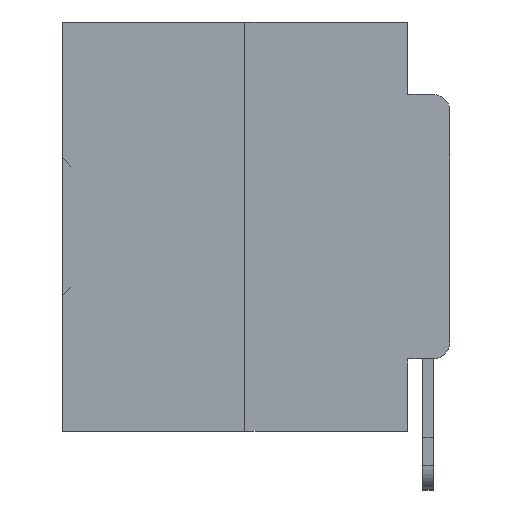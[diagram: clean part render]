
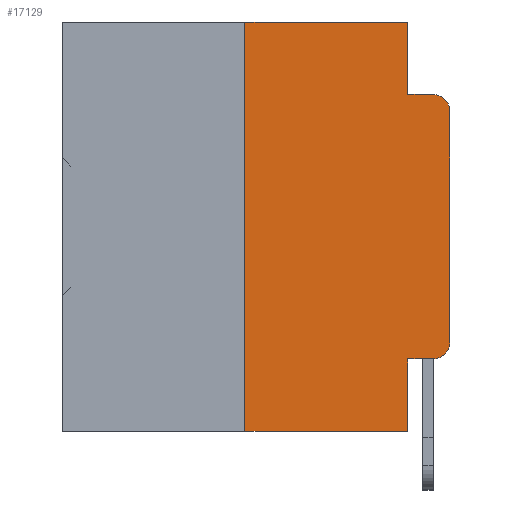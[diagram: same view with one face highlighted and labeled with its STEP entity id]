
A CAD part, left-side view. The second image highlights one B-rep face of the part: STEP entity #17129.
In plain terms, the highlighted planar face has unit normal (-1, 0, 0).
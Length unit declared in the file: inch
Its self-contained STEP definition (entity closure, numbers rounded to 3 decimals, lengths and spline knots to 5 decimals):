
#220 = VERTEX_POINT ( 'NONE', #5546 ) ;
#502 = EDGE_CURVE ( 'NONE', #18418, #23901, #19259, .T. ) ;
#1301 = FACE_OUTER_BOUND ( 'NONE', #3148, .T. ) ;
#2601 = EDGE_CURVE ( 'NONE', #14333, #18418, #7625, .T. ) ;
#2780 = PLANE ( 'NONE',  #14625 ) ;
#2899 = ORIENTED_EDGE ( 'NONE', *, *, #502, .F. ) ;
#3073 = CARTESIAN_POINT ( 'NONE',  ( 0., 0.051, 0. ) ) ;
#3148 = EDGE_LOOP ( 'NONE', ( #19685, #17036, #2899, #5729, #13781, #10040, #9566, #29704, #27873, #22865 ) ) ;
#3236 = CARTESIAN_POINT ( 'NONE',  ( 0., 0.02, -0.0885 ) ) ;
#4004 = VECTOR ( 'NONE', #23836, 39.37008 ) ;
#4418 = VECTOR ( 'NONE', #24037, 39.37008 ) ;
#4629 = EDGE_CURVE ( 'NONE', #12154, #31371, #36298, .T. ) ;
#5309 = DIRECTION ( 'NONE',  ( -1., 0., 0. ) ) ;
#5546 = CARTESIAN_POINT ( 'NONE',  ( 0., 0., -0.1085 ) ) ;
#5729 = ORIENTED_EDGE ( 'NONE', *, *, #2601, .F. ) ;
#5839 = CARTESIAN_POINT ( 'NONE',  ( 0., 0.473, 0. ) ) ;
#6360 = DIRECTION ( 'NONE',  ( 0., -1., 0. ) ) ;
#6972 = CARTESIAN_POINT ( 'NONE',  ( 0., 0.051, -0.5 ) ) ;
#7625 = LINE ( 'NONE', #10183, #15616 ) ;
#8920 = DIRECTION ( 'NONE',  ( 0., 0., -1. ) ) ;
#9404 = CARTESIAN_POINT ( 'NONE',  ( 0., 0., 0. ) ) ;
#9566 = ORIENTED_EDGE ( 'NONE', *, *, #23471, .T. ) ;
#10040 = ORIENTED_EDGE ( 'NONE', *, *, #4629, .F. ) ;
#10183 = CARTESIAN_POINT ( 'NONE',  ( 0., 0.051, 0. ) ) ;
#10333 = DIRECTION ( 'NONE',  ( 0., -1., 0. ) ) ;
#11448 = VECTOR ( 'NONE', #6360, 39.37008 ) ;
#12093 = LINE ( 'NONE', #3073, #4004 ) ;
#12154 = VERTEX_POINT ( 'NONE', #17900 ) ;
#13328 = VECTOR ( 'NONE', #15598, 39.37008 ) ;
#13435 = LINE ( 'NONE', #9404, #4418 ) ;
#13781 = ORIENTED_EDGE ( 'NONE', *, *, #34400, .F. ) ;
#14333 = VERTEX_POINT ( 'NONE', #19620 ) ;
#14571 = VERTEX_POINT ( 'NONE', #32180 ) ;
#14625 = AXIS2_PLACEMENT_3D ( 'NONE', #5839, #26475, #8920 ) ;
#15143 = CARTESIAN_POINT ( 'NONE',  ( 0., 0.02, -0.3915 ) ) ;
#15561 = LINE ( 'NONE', #27823, #30089 ) ;
#15598 = DIRECTION ( 'NONE',  ( 0., -1., 0. ) ) ;
#15616 = VECTOR ( 'NONE', #16480, 39.37008 ) ;
#16480 = DIRECTION ( 'NONE',  ( 0., 0., -1. ) ) ;
#17036 = ORIENTED_EDGE ( 'NONE', *, *, #27150, .T. ) ;
#17129 = ADVANCED_FACE ( 'NONE', ( #1301 ), #2780, .F. ) ;
#17198 = AXIS2_PLACEMENT_3D ( 'NONE', #15143, #35442, #18087 ) ;
#17647 = CARTESIAN_POINT ( 'NONE',  ( 0., 0., -0.3915 ) ) ;
#17900 = CARTESIAN_POINT ( 'NONE',  ( 0., 0.25, -0.5 ) ) ;
#18087 = DIRECTION ( 'NONE',  ( 0., 0., -1. ) ) ;
#18418 = VERTEX_POINT ( 'NONE', #26287 ) ;
#19259 = LINE ( 'NONE', #32983, #11448 ) ;
#19620 = CARTESIAN_POINT ( 'NONE',  ( 0., 0.051, 0. ) ) ;
#19685 = ORIENTED_EDGE ( 'NONE', *, *, #25208, .T. ) ;
#20310 = CARTESIAN_POINT ( 'NONE',  ( 0., 0.25, 0. ) ) ;
#20576 = EDGE_CURVE ( 'NONE', #14571, #29757, #12093, .T. ) ;
#22511 = EDGE_CURVE ( 'NONE', #14571, #24132, #35607, .T. ) ;
#22691 = DIRECTION ( 'NONE',  ( 0., -1., 0. ) ) ;
#22728 = CIRCLE ( 'NONE', #17198, 0.02 ) ;
#22865 = ORIENTED_EDGE ( 'NONE', *, *, #32279, .T. ) ;
#23030 = CARTESIAN_POINT ( 'NONE',  ( 0., 0.02, -0.1085 ) ) ;
#23471 = EDGE_CURVE ( 'NONE', #12154, #29757, #15561, .T. ) ;
#23836 = DIRECTION ( 'NONE',  ( 0., 0., -1. ) ) ;
#23901 = VERTEX_POINT ( 'NONE', #3236 ) ;
#24037 = DIRECTION ( 'NONE',  ( 0., 0., 1. ) ) ;
#24132 = VERTEX_POINT ( 'NONE', #36651 ) ;
#24256 = CARTESIAN_POINT ( 'NONE',  ( 0., 0.473, 0. ) ) ;
#25208 = EDGE_CURVE ( 'NONE', #37679, #220, #13435, .T. ) ;
#25964 = DIRECTION ( 'NONE',  ( 0., 0., -1. ) ) ;
#26287 = CARTESIAN_POINT ( 'NONE',  ( 0., 0.051, -0.0885 ) ) ;
#26335 = CARTESIAN_POINT ( 'NONE',  ( 0., 0.25, 0. ) ) ;
#26458 = CIRCLE ( 'NONE', #35507, 0.02 ) ;
#26475 = DIRECTION ( 'NONE',  ( 1., 0., 0. ) ) ;
#27150 = EDGE_CURVE ( 'NONE', #220, #23901, #26458, .T. ) ;
#27823 = CARTESIAN_POINT ( 'NONE',  ( 0., 0.473, -0.5 ) ) ;
#27873 = ORIENTED_EDGE ( 'NONE', *, *, #22511, .T. ) ;
#28605 = VECTOR ( 'NONE', #29247, 39.37008 ) ;
#29247 = DIRECTION ( 'NONE',  ( 0., 0., 1. ) ) ;
#29704 = ORIENTED_EDGE ( 'NONE', *, *, #20576, .F. ) ;
#29757 = VERTEX_POINT ( 'NONE', #6972 ) ;
#30089 = VECTOR ( 'NONE', #10333, 39.37008 ) ;
#30832 = VECTOR ( 'NONE', #22691, 39.37008 ) ;
#31371 = VERTEX_POINT ( 'NONE', #20310 ) ;
#32180 = CARTESIAN_POINT ( 'NONE',  ( 0., 0.051, -0.4115 ) ) ;
#32279 = EDGE_CURVE ( 'NONE', #24132, #37679, #22728, .T. ) ;
#32646 = LINE ( 'NONE', #24256, #30832 ) ;
#32983 = CARTESIAN_POINT ( 'NONE',  ( 0., 0.051, -0.0885 ) ) ;
#34400 = EDGE_CURVE ( 'NONE', #31371, #14333, #32646, .T. ) ;
#35442 = DIRECTION ( 'NONE',  ( -1., 0., 0. ) ) ;
#35507 = AXIS2_PLACEMENT_3D ( 'NONE', #23030, #5309, #25964 ) ;
#35607 = LINE ( 'NONE', #35892, #13328 ) ;
#35892 = CARTESIAN_POINT ( 'NONE',  ( 0., 0.051, -0.4115 ) ) ;
#36298 = LINE ( 'NONE', #26335, #28605 ) ;
#36651 = CARTESIAN_POINT ( 'NONE',  ( 0., 0.02, -0.4115 ) ) ;
#37679 = VERTEX_POINT ( 'NONE', #17647 ) ;
